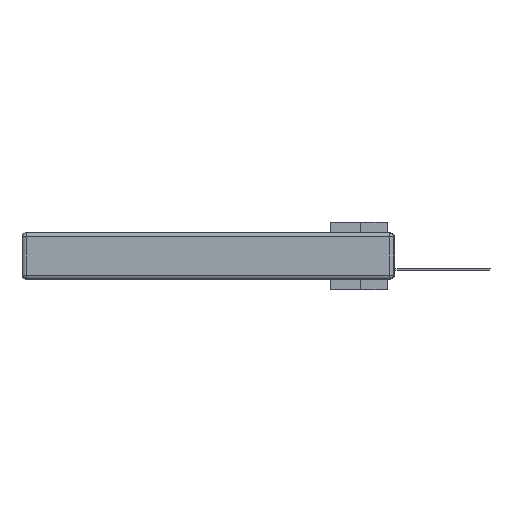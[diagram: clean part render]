
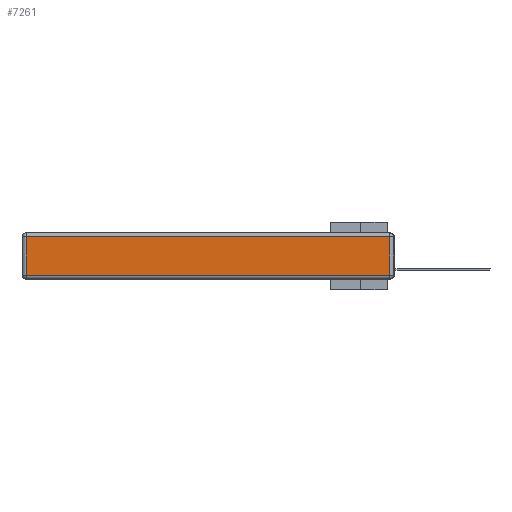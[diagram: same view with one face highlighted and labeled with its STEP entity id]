
A CAD part, left-side view. The second image highlights one B-rep face of the part: STEP entity #7261.
In plain terms, the highlighted planar face has unit normal (-1, 0, 0).
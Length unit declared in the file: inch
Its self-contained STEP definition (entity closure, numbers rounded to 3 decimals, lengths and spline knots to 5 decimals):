
#150 = EDGE_CURVE ( 'NONE', #11366, #14715, #22726, .T. ) ;
#2041 = CARTESIAN_POINT ( 'NONE',  ( 0., 2.72, -0.03 ) ) ;
#2153 = EDGE_LOOP ( 'NONE', ( #23238, #16760, #38114, #14361 ) ) ;
#2428 = EDGE_CURVE ( 'NONE', #25609, #12799, #34822, .T. ) ;
#2790 = VECTOR ( 'NONE', #35578, 39.37008 ) ;
#3414 = CARTESIAN_POINT ( 'NONE',  ( 0., 0.03, -0.03 ) ) ;
#4135 = CARTESIAN_POINT ( 'NONE',  ( 0., 2.75, -0.03 ) ) ;
#5047 = CARTESIAN_POINT ( 'NONE',  ( 0., 0.03, -0.343 ) ) ;
#6011 = DIRECTION ( 'NONE',  ( -1., 0., 0. ) ) ;
#6456 = EDGE_CURVE ( 'NONE', #14715, #25609, #17375, .T. ) ;
#7261 = ADVANCED_FACE ( 'NONE', ( #35390 ), #17376, .T. ) ;
#7456 = DIRECTION ( 'NONE',  ( 0., 1., 0. ) ) ;
#7960 = VECTOR ( 'NONE', #25658, 39.37008 ) ;
#10567 = DIRECTION ( 'NONE',  ( 0., 0., -1. ) ) ;
#11366 = VERTEX_POINT ( 'NONE', #2041 ) ;
#12799 = VERTEX_POINT ( 'NONE', #3414 ) ;
#13467 = AXIS2_PLACEMENT_3D ( 'NONE', #24261, #6011, #23472 ) ;
#14271 = CARTESIAN_POINT ( 'NONE',  ( 0., 2.72, -0.343 ) ) ;
#14361 = ORIENTED_EDGE ( 'NONE', *, *, #150, .T. ) ;
#14504 = VECTOR ( 'NONE', #7456, 39.37008 ) ;
#14715 = VERTEX_POINT ( 'NONE', #15244 ) ;
#15244 = CARTESIAN_POINT ( 'NONE',  ( 0., 2.72, -0.313 ) ) ;
#16760 = ORIENTED_EDGE ( 'NONE', *, *, #2428, .T. ) ;
#17375 = LINE ( 'NONE', #23663, #2790 ) ;
#17376 = PLANE ( 'NONE',  #13467 ) ;
#22726 = LINE ( 'NONE', #14271, #37551 ) ;
#23238 = ORIENTED_EDGE ( 'NONE', *, *, #6456, .T. ) ;
#23472 = DIRECTION ( 'NONE',  ( 0., 0., 1. ) ) ;
#23663 = CARTESIAN_POINT ( 'NONE',  ( 0., 0., -0.313 ) ) ;
#24261 = CARTESIAN_POINT ( 'NONE',  ( 0., 0., -0.343 ) ) ;
#25609 = VERTEX_POINT ( 'NONE', #33104 ) ;
#25658 = DIRECTION ( 'NONE',  ( 0., 0., 1. ) ) ;
#28055 = LINE ( 'NONE', #4135, #14504 ) ;
#32556 = EDGE_CURVE ( 'NONE', #12799, #11366, #28055, .T. ) ;
#33104 = CARTESIAN_POINT ( 'NONE',  ( 0., 0.03, -0.313 ) ) ;
#34822 = LINE ( 'NONE', #5047, #7960 ) ;
#35390 = FACE_OUTER_BOUND ( 'NONE', #2153, .T. ) ;
#35578 = DIRECTION ( 'NONE',  ( 0., -1., 0. ) ) ;
#37551 = VECTOR ( 'NONE', #10567, 39.37008 ) ;
#38114 = ORIENTED_EDGE ( 'NONE', *, *, #32556, .T. ) ;
